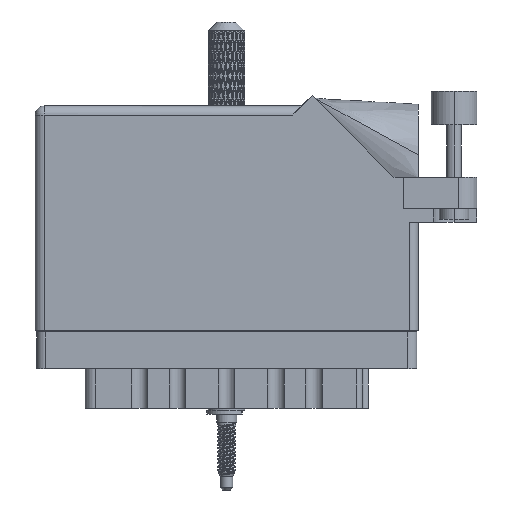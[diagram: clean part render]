
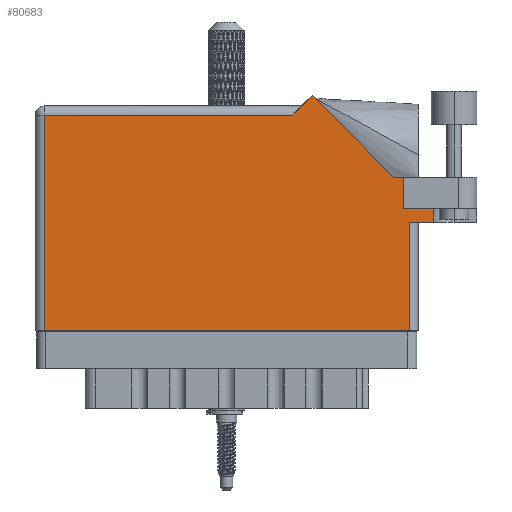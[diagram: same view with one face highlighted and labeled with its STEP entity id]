
A CAD part, front view. The second image highlights one B-rep face of the part: STEP entity #80683.
In plain terms, the highlighted face is planar.
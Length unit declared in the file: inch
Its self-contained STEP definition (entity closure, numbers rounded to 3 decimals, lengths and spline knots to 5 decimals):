
#229 = ORIENTED_EDGE ( 'NONE', *, *, #105985, .T. ) ;
#5661 = CARTESIAN_POINT ( 'NONE',  ( 2.512, 1.044, 0. ) ) ;
#6554 = CARTESIAN_POINT ( 'NONE',  ( 2.612, 0.737, 0. ) ) ;
#7300 = CARTESIAN_POINT ( 'NONE',  ( 0.062, 0., 0. ) ) ;
#7457 = CARTESIAN_POINT ( 'NONE',  ( 1.757, 1.468, 0. ) ) ;
#10544 = ORIENTED_EDGE ( 'NONE', *, *, #73887, .T. ) ;
#10892 = ORIENTED_EDGE ( 'NONE', *, *, #116425, .F. ) ;
#11920 = CARTESIAN_POINT ( 'NONE',  ( 0., 1.468, 0. ) ) ;
#13957 = DIRECTION ( 'NONE',  ( -0.707, 0.707, 0. ) ) ;
#15190 = ORIENTED_EDGE ( 'NONE', *, *, #18259, .F. ) ;
#15725 = CARTESIAN_POINT ( 'NONE',  ( 2.55, 0., 0. ) ) ;
#18259 = EDGE_CURVE ( 'NONE', #43805, #60665, #66734, .T. ) ;
#22930 = ORIENTED_EDGE ( 'NONE', *, *, #47843, .T. ) ;
#27678 = VECTOR ( 'NONE', #89428, 39.37008 ) ;
#29540 = DIRECTION ( 'NONE',  ( -1., 0., 0. ) ) ;
#32396 = ORIENTED_EDGE ( 'NONE', *, *, #75698, .T. ) ;
#32562 = VECTOR ( 'NONE', #42821, 39.37008 ) ;
#34517 = VECTOR ( 'NONE', #13957, 39.37008 ) ;
#34887 = CARTESIAN_POINT ( 'NONE',  ( 2.55, 0.737, 0. ) ) ;
#35753 = EDGE_CURVE ( 'NONE', #50346, #60665, #43015, .T. ) ;
#38905 = ORIENTED_EDGE ( 'NONE', *, *, #58531, .T. ) ;
#39777 = CARTESIAN_POINT ( 'NONE',  ( 2.512, 0.831, 0. ) ) ;
#40881 = EDGE_CURVE ( 'NONE', #109953, #117759, #112012, .T. ) ;
#41894 = DIRECTION ( 'NONE',  ( 0., 0., -1. ) ) ;
#42559 = ORIENTED_EDGE ( 'NONE', *, *, #67564, .T. ) ;
#42821 = DIRECTION ( 'NONE',  ( -0.707, -0.707, 0. ) ) ;
#43015 = LINE ( 'NONE', #6554, #45904 ) ;
#43708 = VECTOR ( 'NONE', #45599, 39.37008 ) ;
#43805 = VERTEX_POINT ( 'NONE', #63232 ) ;
#45599 = DIRECTION ( 'NONE',  ( 0., -1., 0. ) ) ;
#45904 = VECTOR ( 'NONE', #51377, 39.37008 ) ;
#46948 = EDGE_CURVE ( 'NONE', #52623, #50346, #70645, .T. ) ;
#47843 = EDGE_CURVE ( 'NONE', #86413, #103625, #58981, .T. ) ;
#50346 = VERTEX_POINT ( 'NONE', #34887 ) ;
#50920 = CARTESIAN_POINT ( 'NONE',  ( 1.88971, 1.60071, 0. ) ) ;
#51377 = DIRECTION ( 'NONE',  ( 1., 0., 0. ) ) ;
#52114 = LINE ( 'NONE', #107569, #27678 ) ;
#52623 = VERTEX_POINT ( 'NONE', #15725 ) ;
#53648 = CARTESIAN_POINT ( 'NONE',  ( 2.7135, 1.16177, 0. ) ) ;
#55495 = VERTEX_POINT ( 'NONE', #7300 ) ;
#57531 = VECTOR ( 'NONE', #29540, 39.37008 ) ;
#58531 = EDGE_CURVE ( 'NONE', #113750, #86413, #63290, .T. ) ;
#58981 = LINE ( 'NONE', #105122, #34517 ) ;
#59053 = CARTESIAN_POINT ( 'NONE',  ( 0.062, 1.468, 0. ) ) ;
#60663 = CARTESIAN_POINT ( 'NONE',  ( 2.55, 0.737, 0. ) ) ;
#60665 = VERTEX_POINT ( 'NONE', #96188 ) ;
#61851 = LINE ( 'NONE', #62710, #87771 ) ;
#62710 = CARTESIAN_POINT ( 'NONE',  ( 0.062, 0., 0. ) ) ;
#63232 = CARTESIAN_POINT ( 'NONE',  ( 2.7135, 0.831, 0. ) ) ;
#63290 = LINE ( 'NONE', #109166, #57531 ) ;
#66298 = CARTESIAN_POINT ( 'NONE',  ( 2.44642, 1.044, 0. ) ) ;
#66372 = VECTOR ( 'NONE', #88457, 39.37008 ) ;
#66734 = LINE ( 'NONE', #53648, #43708 ) ;
#67564 = EDGE_CURVE ( 'NONE', #55495, #52623, #52114, .T. ) ;
#70645 = LINE ( 'NONE', #60663, #66372 ) ;
#72761 = DIRECTION ( 'NONE',  ( 1., 0., 0. ) ) ;
#73887 = EDGE_CURVE ( 'NONE', #103625, #109953, #106101, .T. ) ;
#75698 = EDGE_CURVE ( 'NONE', #87471, #113750, #117353, .T. ) ;
#76983 = PLANE ( 'NONE',  #103722 ) ;
#77239 = DIRECTION ( 'NONE',  ( -1., 0., 0. ) ) ;
#77901 = ORIENTED_EDGE ( 'NONE', *, *, #40881, .T. ) ;
#79062 = CARTESIAN_POINT ( 'NONE',  ( 1.819, 1.53, 0. ) ) ;
#79641 = VECTOR ( 'NONE', #72761, 39.37008 ) ;
#80013 = DIRECTION ( 'NONE',  ( 0., -1., 0. ) ) ;
#80551 = EDGE_LOOP ( 'NONE', ( #42559, #97726, #102636, #15190, #10892, #32396, #38905, #22930, #10544, #77901, #229 ) ) ;
#80683 = ADVANCED_FACE ( 'NONE', ( #104494 ), #76983, .F. ) ;
#86413 = VERTEX_POINT ( 'NONE', #66298 ) ;
#86864 = LINE ( 'NONE', #91780, #79641 ) ;
#87471 = VERTEX_POINT ( 'NONE', #110794 ) ;
#87771 = VECTOR ( 'NONE', #80013, 39.37008 ) ;
#88457 = DIRECTION ( 'NONE',  ( 0., 1., 0. ) ) ;
#89428 = DIRECTION ( 'NONE',  ( 1., 0., 0. ) ) ;
#91780 = CARTESIAN_POINT ( 'NONE',  ( 2.512, 0.831, 0. ) ) ;
#96188 = CARTESIAN_POINT ( 'NONE',  ( 2.7135, 0.737, 0. ) ) ;
#97558 = CARTESIAN_POINT ( 'NONE',  ( 0., 1.53, 0. ) ) ;
#97726 = ORIENTED_EDGE ( 'NONE', *, *, #46948, .T. ) ;
#102636 = ORIENTED_EDGE ( 'NONE', *, *, #35753, .T. ) ;
#103625 = VERTEX_POINT ( 'NONE', #50920 ) ;
#103722 = AXIS2_PLACEMENT_3D ( 'NONE', #97558, #41894, #105634 ) ;
#104494 = FACE_OUTER_BOUND ( 'NONE', #80551, .T. ) ;
#105122 = CARTESIAN_POINT ( 'NONE',  ( 2.44642, 1.044, 0. ) ) ;
#105634 = DIRECTION ( 'NONE',  ( -1., 0., 0. ) ) ;
#105985 = EDGE_CURVE ( 'NONE', #117759, #55495, #61851, .T. ) ;
#106101 = LINE ( 'NONE', #79062, #32562 ) ;
#107569 = CARTESIAN_POINT ( 'NONE',  ( 0., 0., 0. ) ) ;
#107716 = VECTOR ( 'NONE', #77239, 39.37008 ) ;
#109166 = CARTESIAN_POINT ( 'NONE',  ( 3.012, 1.044, 0. ) ) ;
#109953 = VERTEX_POINT ( 'NONE', #7457 ) ;
#110794 = CARTESIAN_POINT ( 'NONE',  ( 2.512, 0.831, 0. ) ) ;
#112012 = LINE ( 'NONE', #11920, #107716 ) ;
#112799 = DIRECTION ( 'NONE',  ( 0., 1., 0. ) ) ;
#113750 = VERTEX_POINT ( 'NONE', #5661 ) ;
#115961 = VECTOR ( 'NONE', #112799, 39.37008 ) ;
#116425 = EDGE_CURVE ( 'NONE', #87471, #43805, #86864, .T. ) ;
#117353 = LINE ( 'NONE', #39777, #115961 ) ;
#117759 = VERTEX_POINT ( 'NONE', #59053 ) ;
